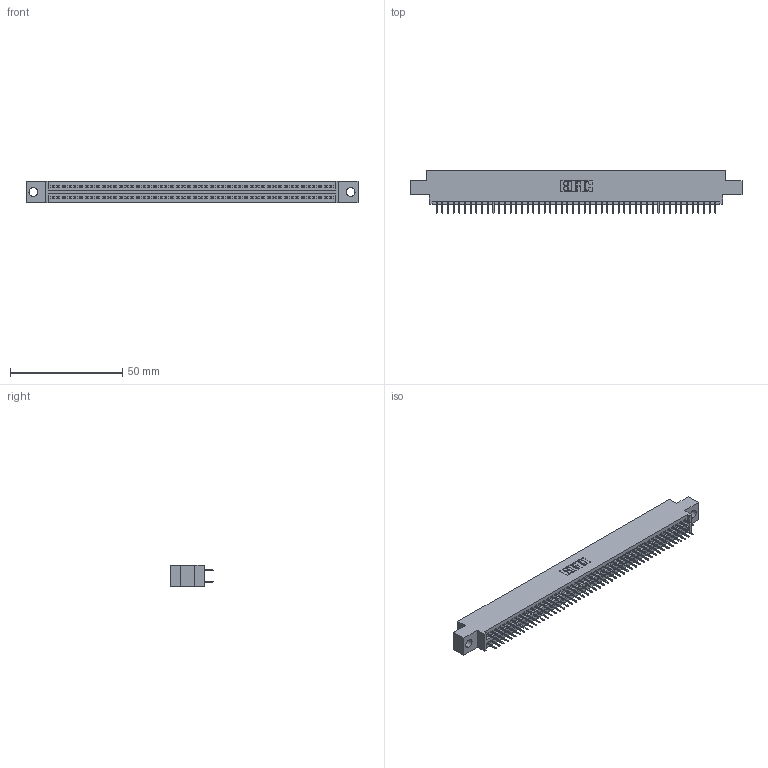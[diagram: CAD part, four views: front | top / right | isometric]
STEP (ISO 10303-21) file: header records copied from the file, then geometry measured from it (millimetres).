
FILE_DESCRIPTION (( 'STEP AP203' ), '1' );
FILE_NAME ('395-100-524-804.STEP', '2021-06-17T15:02:48', ( '' ), ( '' ), 'SwSTEP 2.0', 'SolidWorks 2020', '' );
FILE_SCHEMA (( 'CONFIG_CONTROL_DESIGN' ));
Length unit declared in the file: inch
Products named in the file (3): 395-100-524-804; 345 Part_0.170 Offset - 0.156 Dia-TI; 345-292-001_345-293-124
Assembly tree (101 placements, depth 2):
  395-100-524-804
    345 Part_0.170 Offset - 0.156 Dia-TI
    345-292-001_345-293-124  x100
Bounding box: 148.21 x 19.35 x 9.4 mm (x, y, z)
Volume: 14100.8 mm3; surface area: 20593.8 mm2
Topology: 101 solids, 101 shells, 5544 faces, 15689 edges, 10058 vertices
Faces by surface type: plane 3998, cylinder 1546
Entity records: 38779 total; most frequent: CARTESIAN_POINT 6498, ORIENTED_EDGE 6430, DIRECTION 5719, EDGE_CURVE 3215, LINE 2887, VECTOR 2887, VERTEX_POINT 2138, AXIS2_PLACEMENT_3D 1416
